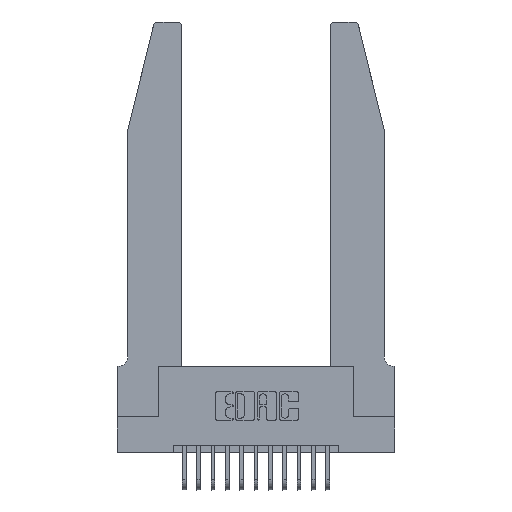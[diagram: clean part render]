
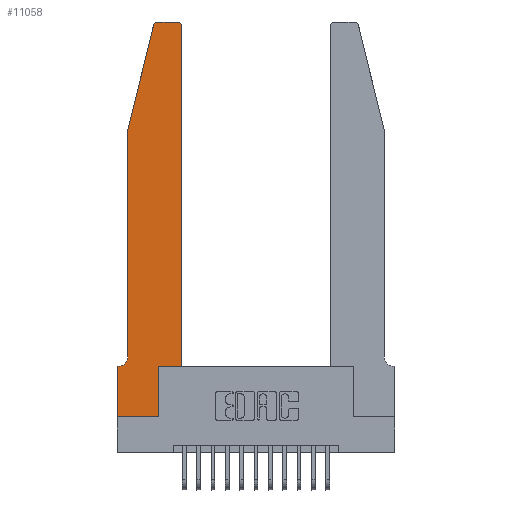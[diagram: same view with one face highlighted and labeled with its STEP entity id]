
A CAD part, top view. The second image highlights one B-rep face of the part: STEP entity #11058.
In plain terms, the highlighted planar face has unit normal (0, 0, 1).
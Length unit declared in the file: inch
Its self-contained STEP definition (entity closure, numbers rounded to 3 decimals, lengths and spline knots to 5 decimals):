
#281 = ORIENTED_EDGE ( 'NONE', *, *, #6950, .T. ) ;
#408 = DIRECTION ( 'NONE',  ( -1., 0., 0. ) ) ;
#711 = ORIENTED_EDGE ( 'NONE', *, *, #5072, .T. ) ;
#743 = LINE ( 'NONE', #7276, #7615 ) ;
#948 = ORIENTED_EDGE ( 'NONE', *, *, #12073, .T. ) ;
#1135 = DIRECTION ( 'NONE',  ( 0., -1., 0. ) ) ;
#2293 = VERTEX_POINT ( 'NONE', #6730 ) ;
#2344 = DIRECTION ( 'NONE',  ( 0., -1., 0. ) ) ;
#2394 = DIRECTION ( 'NONE',  ( 0., 0., -1. ) ) ;
#2490 = DIRECTION ( 'NONE',  ( 1., 0., 0. ) ) ;
#2609 = VERTEX_POINT ( 'NONE', #13700 ) ;
#2794 = EDGE_CURVE ( 'NONE', #13722, #2837, #16408, .T. ) ;
#2837 = VERTEX_POINT ( 'NONE', #16126 ) ;
#3176 = EDGE_CURVE ( 'NONE', #2293, #3937, #14992, .T. ) ;
#3205 = EDGE_LOOP ( 'NONE', ( #12566, #281, #711, #15385, #12373, #9277, #16588, #10101, #3802, #948, #11763, #15615 ) ) ;
#3707 = CARTESIAN_POINT ( 'NONE',  ( 0., 0., 0.37 ) ) ;
#3802 = ORIENTED_EDGE ( 'NONE', *, *, #12342, .T. ) ;
#3937 = VERTEX_POINT ( 'NONE', #3707 ) ;
#3971 = CARTESIAN_POINT ( 'NONE',  ( 0., 0.35, 0.37 ) ) ;
#4404 = DIRECTION ( 'NONE',  ( 0., 1., 0. ) ) ;
#4733 = DIRECTION ( 'NONE',  ( 0., 0., 1. ) ) ;
#4785 = VERTEX_POINT ( 'NONE', #8099 ) ;
#4910 = VERTEX_POINT ( 'NONE', #16481 ) ;
#4932 = LINE ( 'NONE', #14979, #7625 ) ;
#4990 = LINE ( 'NONE', #8268, #8107 ) ;
#5072 = EDGE_CURVE ( 'NONE', #4910, #13722, #9596, .T. ) ;
#5077 = DIRECTION ( 'NONE',  ( -0.239, -0.971, 0. ) ) ;
#5370 = DIRECTION ( 'NONE',  ( 1., 0., 0. ) ) ;
#5422 = EDGE_CURVE ( 'NONE', #3937, #9213, #13903, .T. ) ;
#5639 = VECTOR ( 'NONE', #5077, 39.37008 ) ;
#5745 = CARTESIAN_POINT ( 'NONE',  ( 0., 0., 0.37 ) ) ;
#6129 = VERTEX_POINT ( 'NONE', #10568 ) ;
#6216 = LINE ( 'NONE', #7642, #15450 ) ;
#6693 = EDGE_CURVE ( 'NONE', #9533, #2293, #6216, .T. ) ;
#6730 = CARTESIAN_POINT ( 'NONE',  ( 0., 0.35, 0.37 ) ) ;
#6842 = DIRECTION ( 'NONE',  ( 0., 0., 1. ) ) ;
#6889 = VECTOR ( 'NONE', #7588, 39.37008 ) ;
#6950 = EDGE_CURVE ( 'NONE', #9124, #4910, #14851, .T. ) ;
#7109 = CARTESIAN_POINT ( 'NONE',  ( 0.0055, 0.35, 0.37 ) ) ;
#7276 = CARTESIAN_POINT ( 'NONE',  ( 0.2605, 2.75, 0.37 ) ) ;
#7431 = LINE ( 'NONE', #15728, #10555 ) ;
#7533 = VERTEX_POINT ( 'NONE', #12381 ) ;
#7588 = DIRECTION ( 'NONE',  ( 1., 0., 0. ) ) ;
#7615 = VECTOR ( 'NONE', #408, 39.37008 ) ;
#7619 = EDGE_CURVE ( 'NONE', #7533, #9124, #743, .T. ) ;
#7625 = VECTOR ( 'NONE', #4404, 39.37008 ) ;
#7642 = CARTESIAN_POINT ( 'NONE',  ( 0.0755, 0.35, 0.37 ) ) ;
#8099 = CARTESIAN_POINT ( 'NONE',  ( 0.4505, 2.72, 0.37 ) ) ;
#8107 = VECTOR ( 'NONE', #16104, 39.37008 ) ;
#8268 = CARTESIAN_POINT ( 'NONE',  ( 0.4505, 0.35, 0.37 ) ) ;
#8919 = CARTESIAN_POINT ( 'NONE',  ( 0.2865, 0., 0.37 ) ) ;
#8932 = CARTESIAN_POINT ( 'NONE',  ( 0.0755, 2., 0.37 ) ) ;
#9124 = VERTEX_POINT ( 'NONE', #12678 ) ;
#9213 = VERTEX_POINT ( 'NONE', #8919 ) ;
#9277 = ORIENTED_EDGE ( 'NONE', *, *, #6693, .T. ) ;
#9466 = AXIS2_PLACEMENT_3D ( 'NONE', #12688, #4733, #13992 ) ;
#9533 = VERTEX_POINT ( 'NONE', #7109 ) ;
#9596 = LINE ( 'NONE', #14266, #5639 ) ;
#10101 = ORIENTED_EDGE ( 'NONE', *, *, #5422, .T. ) ;
#10454 = CARTESIAN_POINT ( 'NONE',  ( 0.0055, 0.42, 0.37 ) ) ;
#10555 = VECTOR ( 'NONE', #2490, 39.37008 ) ;
#10568 = CARTESIAN_POINT ( 'NONE',  ( 0.4505, 0.35, 0.37 ) ) ;
#11058 = ADVANCED_FACE ( 'NONE', ( #11833 ), #11981, .T. ) ;
#11391 = EDGE_CURVE ( 'NONE', #2837, #9533, #17264, .T. ) ;
#11474 = CARTESIAN_POINT ( 'NONE',  ( 0.0755, 2., 0.37 ) ) ;
#11763 = ORIENTED_EDGE ( 'NONE', *, *, #16639, .T. ) ;
#11781 = DIRECTION ( 'NONE',  ( -1., 0., 0. ) ) ;
#11833 = FACE_OUTER_BOUND ( 'NONE', #3205, .T. ) ;
#11981 = PLANE ( 'NONE',  #15841 ) ;
#12073 = EDGE_CURVE ( 'NONE', #2609, #6129, #7431, .T. ) ;
#12342 = EDGE_CURVE ( 'NONE', #9213, #2609, #4932, .T. ) ;
#12373 = ORIENTED_EDGE ( 'NONE', *, *, #11391, .T. ) ;
#12381 = CARTESIAN_POINT ( 'NONE',  ( 0.4205, 2.75, 0.37 ) ) ;
#12566 = ORIENTED_EDGE ( 'NONE', *, *, #7619, .T. ) ;
#12678 = CARTESIAN_POINT ( 'NONE',  ( 0.284, 2.75, 0.37 ) ) ;
#12688 = CARTESIAN_POINT ( 'NONE',  ( 0.4205, 2.72, 0.37 ) ) ;
#12930 = AXIS2_PLACEMENT_3D ( 'NONE', #10454, #2394, #11781 ) ;
#13304 = DIRECTION ( 'NONE',  ( 0., 0., 1. ) ) ;
#13411 = VECTOR ( 'NONE', #1135, 39.37008 ) ;
#13700 = CARTESIAN_POINT ( 'NONE',  ( 0.2865, 0.35, 0.37 ) ) ;
#13722 = VERTEX_POINT ( 'NONE', #8932 ) ;
#13903 = LINE ( 'NONE', #15390, #6889 ) ;
#13992 = DIRECTION ( 'NONE',  ( 1., 0., 0. ) ) ;
#14266 = CARTESIAN_POINT ( 'NONE',  ( 0.0755, 2., 0.37 ) ) ;
#14724 = CARTESIAN_POINT ( 'NONE',  ( 0.284, 2.72, 0.37 ) ) ;
#14851 = CIRCLE ( 'NONE', #16308, 0.03 ) ;
#14979 = CARTESIAN_POINT ( 'NONE',  ( 0.2865, 0.35, 0.37 ) ) ;
#14992 = LINE ( 'NONE', #5745, #17196 ) ;
#15385 = ORIENTED_EDGE ( 'NONE', *, *, #2794, .T. ) ;
#15390 = CARTESIAN_POINT ( 'NONE',  ( 0., 0., 0.37 ) ) ;
#15450 = VECTOR ( 'NONE', #15505, 39.37008 ) ;
#15505 = DIRECTION ( 'NONE',  ( -1., 0., 0. ) ) ;
#15615 = ORIENTED_EDGE ( 'NONE', *, *, #15749, .T. ) ;
#15728 = CARTESIAN_POINT ( 'NONE',  ( 0.4505, 0.35, 0.37 ) ) ;
#15749 = EDGE_CURVE ( 'NONE', #4785, #7533, #15933, .T. ) ;
#15841 = AXIS2_PLACEMENT_3D ( 'NONE', #3971, #13304, #5370 ) ;
#15933 = CIRCLE ( 'NONE', #9466, 0.03 ) ;
#16014 = DIRECTION ( 'NONE',  ( 1., 0., 0. ) ) ;
#16104 = DIRECTION ( 'NONE',  ( 0., 1., 0. ) ) ;
#16126 = CARTESIAN_POINT ( 'NONE',  ( 0.0755, 0.42, 0.37 ) ) ;
#16308 = AXIS2_PLACEMENT_3D ( 'NONE', #14724, #6842, #16014 ) ;
#16408 = LINE ( 'NONE', #11474, #13411 ) ;
#16481 = CARTESIAN_POINT ( 'NONE',  ( 0.25487, 2.72718, 0.37 ) ) ;
#16588 = ORIENTED_EDGE ( 'NONE', *, *, #3176, .T. ) ;
#16639 = EDGE_CURVE ( 'NONE', #6129, #4785, #4990, .T. ) ;
#17196 = VECTOR ( 'NONE', #2344, 39.37008 ) ;
#17264 = CIRCLE ( 'NONE', #12930, 0.07 ) ;
